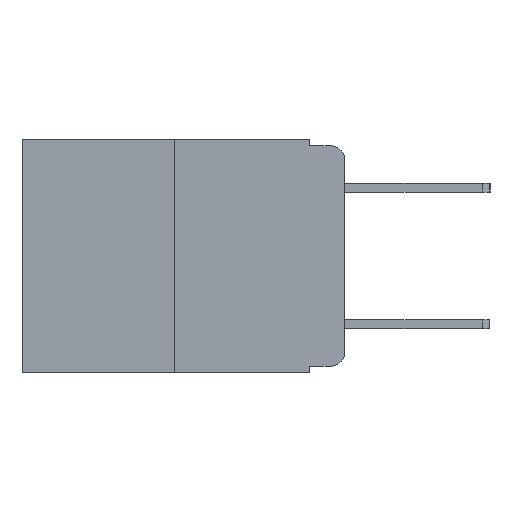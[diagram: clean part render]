
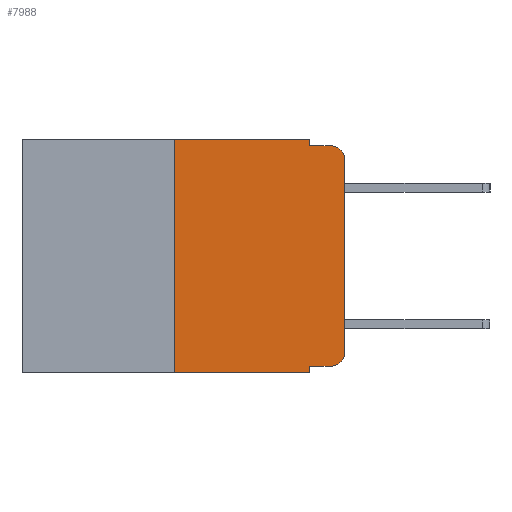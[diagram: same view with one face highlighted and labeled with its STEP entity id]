
A CAD part, left-side view. The second image highlights one B-rep face of the part: STEP entity #7988.
In plain terms, the highlighted planar face has unit normal (-1, 0, 0).
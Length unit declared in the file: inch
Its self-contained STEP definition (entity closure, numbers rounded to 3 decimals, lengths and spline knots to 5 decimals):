
#536 = VERTEX_POINT ( 'NONE', #11040 ) ;
#763 = DIRECTION ( 'NONE',  ( 0., 0., 1. ) ) ;
#844 = CARTESIAN_POINT ( 'NONE',  ( 0., 0.051, 0. ) ) ;
#993 = CARTESIAN_POINT ( 'NONE',  ( 0., 0.473, 0. ) ) ;
#1115 = DIRECTION ( 'NONE',  ( 0., -1., 0. ) ) ;
#1156 = AXIS2_PLACEMENT_3D ( 'NONE', #11660, #6287, #12531 ) ;
#1263 = DIRECTION ( 'NONE',  ( 0., -1., 0. ) ) ;
#1585 = PLANE ( 'NONE',  #2753 ) ;
#1719 = LINE ( 'NONE', #8450, #8789 ) ;
#1725 = CARTESIAN_POINT ( 'NONE',  ( 0., 0.051, 0. ) ) ;
#1910 = VERTEX_POINT ( 'NONE', #10163 ) ;
#2053 = CARTESIAN_POINT ( 'NONE',  ( 0., 0.25, 0. ) ) ;
#2570 = EDGE_CURVE ( 'NONE', #7987, #5036, #1719, .T. ) ;
#2574 = EDGE_CURVE ( 'NONE', #8520, #7987, #6660, .T. ) ;
#2575 = EDGE_CURVE ( 'NONE', #1910, #5036, #6363, .T. ) ;
#2701 = EDGE_CURVE ( 'NONE', #536, #1910, #6209, .T. ) ;
#2753 = AXIS2_PLACEMENT_3D ( 'NONE', #8663, #2830, #9569 ) ;
#2824 = VECTOR ( 'NONE', #8755, 39.37008 ) ;
#2830 = DIRECTION ( 'NONE',  ( 1., 0., 0. ) ) ;
#2902 = ORIENTED_EDGE ( 'NONE', *, *, #2575, .T. ) ;
#3065 = DIRECTION ( 'NONE',  ( 0., 0., 1. ) ) ;
#3122 = EDGE_CURVE ( 'NONE', #10423, #8520, #12076, .T. ) ;
#3144 = EDGE_CURVE ( 'NONE', #6778, #6593, #4161, .T. ) ;
#3470 = DIRECTION ( 'NONE',  ( 0., -1., 0. ) ) ;
#3666 = CARTESIAN_POINT ( 'NONE',  ( 0., 0.051, 0. ) ) ;
#3701 = DIRECTION ( 'NONE',  ( -1., 0., 0. ) ) ;
#3711 = VECTOR ( 'NONE', #11998, 39.37008 ) ;
#3797 = VECTOR ( 'NONE', #4010, 39.37008 ) ;
#3851 = CARTESIAN_POINT ( 'NONE',  ( 0., 0.051, -0.01 ) ) ;
#3883 = EDGE_CURVE ( 'NONE', #9301, #6593, #10142, .T. ) ;
#4010 = DIRECTION ( 'NONE',  ( 0., -1., 0. ) ) ;
#4161 = LINE ( 'NONE', #12736, #11253 ) ;
#4227 = EDGE_LOOP ( 'NONE', ( #10194, #2902, #8109, #10481, #5948, #10765, #11030, #11298, #6827, #11585 ) ) ;
#4452 = CARTESIAN_POINT ( 'NONE',  ( 0., 0.25, -0.343 ) ) ;
#4801 = VECTOR ( 'NONE', #3470, 39.37008 ) ;
#4873 = EDGE_CURVE ( 'NONE', #9301, #10467, #9711, .T. ) ;
#5036 = VERTEX_POINT ( 'NONE', #12563 ) ;
#5271 = CARTESIAN_POINT ( 'NONE',  ( 0., 0.051, -0.333 ) ) ;
#5948 = ORIENTED_EDGE ( 'NONE', *, *, #3122, .F. ) ;
#6197 = VECTOR ( 'NONE', #763, 39.37008 ) ;
#6209 = LINE ( 'NONE', #12324, #8366 ) ;
#6287 = DIRECTION ( 'NONE',  ( -1., 0., 0. ) ) ;
#6363 = CIRCLE ( 'NONE', #9658, 0.02 ) ;
#6541 = CARTESIAN_POINT ( 'NONE',  ( 0., 0.25, 0. ) ) ;
#6545 = EDGE_CURVE ( 'NONE', #10467, #536, #10228, .T. ) ;
#6593 = VERTEX_POINT ( 'NONE', #10824 ) ;
#6660 = LINE ( 'NONE', #3666, #3711 ) ;
#6778 = VERTEX_POINT ( 'NONE', #4452 ) ;
#6827 = ORIENTED_EDGE ( 'NONE', *, *, #4873, .T. ) ;
#7904 = CARTESIAN_POINT ( 'NONE',  ( 0., 0.051, -0.333 ) ) ;
#7987 = VERTEX_POINT ( 'NONE', #3851 ) ;
#7988 = ADVANCED_FACE ( 'NONE', ( #12025 ), #1585, .F. ) ;
#8109 = ORIENTED_EDGE ( 'NONE', *, *, #2570, .F. ) ;
#8366 = VECTOR ( 'NONE', #3065, 39.37008 ) ;
#8450 = CARTESIAN_POINT ( 'NONE',  ( 0., 0.051, -0.01 ) ) ;
#8520 = VERTEX_POINT ( 'NONE', #844 ) ;
#8641 = LINE ( 'NONE', #2053, #6197 ) ;
#8663 = CARTESIAN_POINT ( 'NONE',  ( 0., 0.473, 0. ) ) ;
#8755 = DIRECTION ( 'NONE',  ( 0., 0., -1. ) ) ;
#8789 = VECTOR ( 'NONE', #1263, 39.37008 ) ;
#9301 = VERTEX_POINT ( 'NONE', #5271 ) ;
#9386 = CARTESIAN_POINT ( 'NONE',  ( 0., 0.02, -0.03 ) ) ;
#9569 = DIRECTION ( 'NONE',  ( 0., 0., -1. ) ) ;
#9658 = AXIS2_PLACEMENT_3D ( 'NONE', #9386, #3701, #10268 ) ;
#9711 = LINE ( 'NONE', #7904, #3797 ) ;
#10142 = LINE ( 'NONE', #1725, #2824 ) ;
#10163 = CARTESIAN_POINT ( 'NONE',  ( 0., 0., -0.03 ) ) ;
#10194 = ORIENTED_EDGE ( 'NONE', *, *, #2701, .T. ) ;
#10228 = CIRCLE ( 'NONE', #1156, 0.02 ) ;
#10268 = DIRECTION ( 'NONE',  ( 0., 0., -1. ) ) ;
#10423 = VERTEX_POINT ( 'NONE', #6541 ) ;
#10467 = VERTEX_POINT ( 'NONE', #11937 ) ;
#10481 = ORIENTED_EDGE ( 'NONE', *, *, #2574, .F. ) ;
#10765 = ORIENTED_EDGE ( 'NONE', *, *, #12403, .F. ) ;
#10824 = CARTESIAN_POINT ( 'NONE',  ( 0., 0.051, -0.343 ) ) ;
#11030 = ORIENTED_EDGE ( 'NONE', *, *, #3144, .T. ) ;
#11040 = CARTESIAN_POINT ( 'NONE',  ( 0., 0., -0.313 ) ) ;
#11253 = VECTOR ( 'NONE', #1115, 39.37008 ) ;
#11298 = ORIENTED_EDGE ( 'NONE', *, *, #3883, .F. ) ;
#11585 = ORIENTED_EDGE ( 'NONE', *, *, #6545, .T. ) ;
#11660 = CARTESIAN_POINT ( 'NONE',  ( 0., 0.02, -0.313 ) ) ;
#11937 = CARTESIAN_POINT ( 'NONE',  ( 0., 0.02, -0.333 ) ) ;
#11998 = DIRECTION ( 'NONE',  ( 0., 0., -1. ) ) ;
#12025 = FACE_OUTER_BOUND ( 'NONE', #4227, .T. ) ;
#12076 = LINE ( 'NONE', #993, #4801 ) ;
#12324 = CARTESIAN_POINT ( 'NONE',  ( 0., 0., 0. ) ) ;
#12403 = EDGE_CURVE ( 'NONE', #6778, #10423, #8641, .T. ) ;
#12531 = DIRECTION ( 'NONE',  ( 0., 0., -1. ) ) ;
#12563 = CARTESIAN_POINT ( 'NONE',  ( 0., 0.02, -0.01 ) ) ;
#12736 = CARTESIAN_POINT ( 'NONE',  ( 0., 0.473, -0.343 ) ) ;
